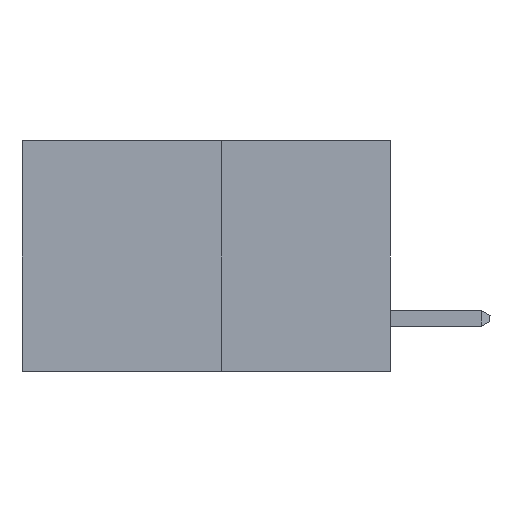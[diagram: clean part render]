
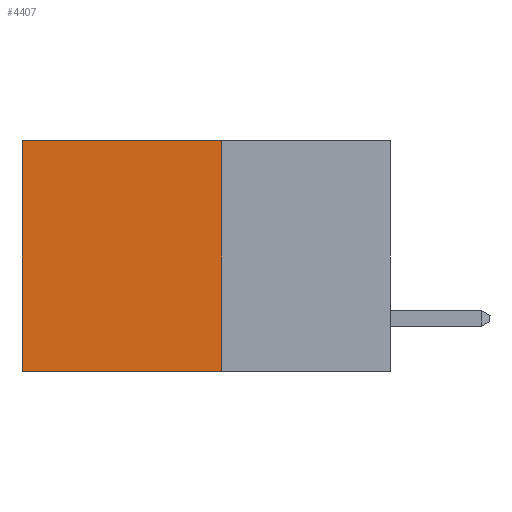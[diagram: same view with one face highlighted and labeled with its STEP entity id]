
A CAD part, left-side view. The second image highlights one B-rep face of the part: STEP entity #4407.
In plain terms, the highlighted planar face has unit normal (-1, 0, 0).
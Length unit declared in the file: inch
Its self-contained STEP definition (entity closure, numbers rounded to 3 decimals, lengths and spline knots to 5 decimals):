
#77 = ORIENTED_EDGE ( 'NONE', *, *, #2131, .F. ) ;
#1205 = CARTESIAN_POINT ( 'NONE',  ( 0.277, 0.59, 0. ) ) ;
#1965 = EDGE_LOOP ( 'NONE', ( #20009, #12929, #77, #13922 ) ) ;
#2131 = EDGE_CURVE ( 'NONE', #19407, #18286, #21189, .T. ) ;
#2328 = DIRECTION ( 'NONE',  ( 0., 1., 0. ) ) ;
#3234 = CARTESIAN_POINT ( 'NONE',  ( 0.277, 0.27, -0.37 ) ) ;
#3400 = VECTOR ( 'NONE', #2328, 39.37008 ) ;
#3746 = LINE ( 'NONE', #17290, #19775 ) ;
#4142 = AXIS2_PLACEMENT_3D ( 'NONE', #15592, #15336, #15329 ) ;
#4407 = ADVANCED_FACE ( 'NONE', ( #16227 ), #15666, .F. ) ;
#5608 = CARTESIAN_POINT ( 'NONE',  ( 0.277, 0.27, -0.37 ) ) ;
#6756 = CARTESIAN_POINT ( 'NONE',  ( 0.277, 0.59, -0.37 ) ) ;
#7393 = LINE ( 'NONE', #6756, #12893 ) ;
#8161 = VECTOR ( 'NONE', #8494, 39.37008 ) ;
#8299 = VERTEX_POINT ( 'NONE', #1205 ) ;
#8425 = LINE ( 'NONE', #5608, #3400 ) ;
#8494 = DIRECTION ( 'NONE',  ( 0., 0., -1. ) ) ;
#9687 = VERTEX_POINT ( 'NONE', #19006 ) ;
#11673 = CARTESIAN_POINT ( 'NONE',  ( 0.277, 0.27, 0. ) ) ;
#12893 = VECTOR ( 'NONE', #16635, 39.37008 ) ;
#12929 = ORIENTED_EDGE ( 'NONE', *, *, #14473, .F. ) ;
#13922 = ORIENTED_EDGE ( 'NONE', *, *, #20616, .T. ) ;
#14473 = EDGE_CURVE ( 'NONE', #18286, #9687, #8425, .T. ) ;
#15329 = DIRECTION ( 'NONE',  ( 0., 0., -1. ) ) ;
#15336 = DIRECTION ( 'NONE',  ( 1., 0., 0. ) ) ;
#15592 = CARTESIAN_POINT ( 'NONE',  ( 0.277, 0.27, -0.37 ) ) ;
#15666 = PLANE ( 'NONE',  #4142 ) ;
#16130 = EDGE_CURVE ( 'NONE', #8299, #9687, #7393, .T. ) ;
#16227 = FACE_OUTER_BOUND ( 'NONE', #1965, .T. ) ;
#16635 = DIRECTION ( 'NONE',  ( 0., 0., -1. ) ) ;
#17290 = CARTESIAN_POINT ( 'NONE',  ( 0.277, 0.27, 0. ) ) ;
#18286 = VERTEX_POINT ( 'NONE', #20214 ) ;
#18933 = DIRECTION ( 'NONE',  ( 0., 1., 0. ) ) ;
#19006 = CARTESIAN_POINT ( 'NONE',  ( 0.277, 0.59, -0.37 ) ) ;
#19407 = VERTEX_POINT ( 'NONE', #11673 ) ;
#19775 = VECTOR ( 'NONE', #18933, 39.37008 ) ;
#20009 = ORIENTED_EDGE ( 'NONE', *, *, #16130, .T. ) ;
#20214 = CARTESIAN_POINT ( 'NONE',  ( 0.277, 0.27, -0.37 ) ) ;
#20616 = EDGE_CURVE ( 'NONE', #19407, #8299, #3746, .T. ) ;
#21189 = LINE ( 'NONE', #3234, #8161 ) ;
